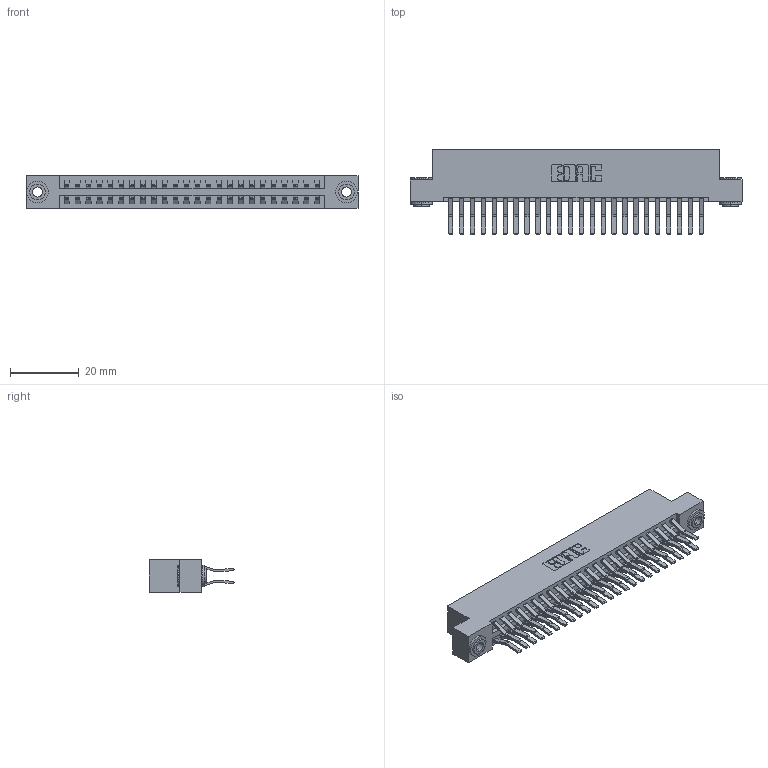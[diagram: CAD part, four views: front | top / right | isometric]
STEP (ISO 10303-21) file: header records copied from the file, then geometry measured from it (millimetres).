
FILE_DESCRIPTION (( 'STEP AP203' ), '1' );
FILE_NAME ('346-048-560-203.STEP', '2018-08-25T11:18:20', ( '' ), ( '' ), 'SwSTEP 2.0', 'SolidWorks 2016', '' );
FILE_SCHEMA (( 'CONFIG_CONTROL_DESIGN' ));
Length unit declared in the file: inch
Products named in the file (4): 346 Part_Flush Mounting Lugs - 0.156 Dia-TH; 345-292-001_560 Tail; 345-250-002_345-250-002-102; 346-048-560-203
Assembly tree (51 placements, depth 2):
  346-048-560-203
    346 Part_Flush Mounting Lugs - 0.156 Dia-TH
    345-292-001_560 Tail  x48
    345-250-002_345-250-002-102  x2
Bounding box: 96.77 x 24.78 x 9.4 mm (x, y, z)
Volume: 9630.9 mm3; surface area: 14008.9 mm2
Topology: 51 solids, 51 shells, 2752 faces, 8133 edges, 5354 vertices
Faces by surface type: plane 1766, cylinder 978, cone 8
Entity records: 18824 total; most frequent: CARTESIAN_POINT 3103, ORIENTED_EDGE 3030, DIRECTION 2821, EDGE_CURVE 1515, LINE 1259, VECTOR 1259, VERTEX_POINT 1006, AXIS2_PLACEMENT_3D 781
